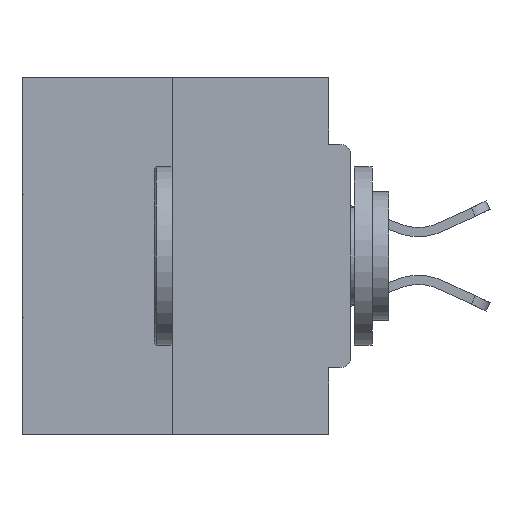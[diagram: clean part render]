
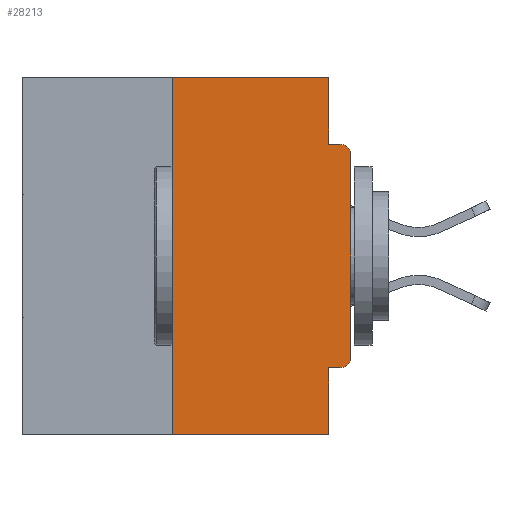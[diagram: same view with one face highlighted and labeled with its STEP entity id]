
A CAD part, left-side view. The second image highlights one B-rep face of the part: STEP entity #28213.
In plain terms, the highlighted planar face has unit normal (-1, 0, 0).
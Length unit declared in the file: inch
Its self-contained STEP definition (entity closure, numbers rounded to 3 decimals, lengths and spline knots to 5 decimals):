
#609 = VERTEX_POINT ( 'NONE', #28277 ) ;
#995 = LINE ( 'NONE', #14118, #32650 ) ;
#1202 = ORIENTED_EDGE ( 'NONE', *, *, #29794, .T. ) ;
#1349 = ORIENTED_EDGE ( 'NONE', *, *, #2727, .T. ) ;
#1656 = LINE ( 'NONE', #17639, #36566 ) ;
#1815 = CARTESIAN_POINT ( 'NONE',  ( 0., 0.25, 0. ) ) ;
#2324 = CARTESIAN_POINT ( 'NONE',  ( 0., 0.015, -0.4065 ) ) ;
#2508 = PLANE ( 'NONE',  #12070 ) ;
#2518 = VERTEX_POINT ( 'NONE', #1815 ) ;
#2727 = EDGE_CURVE ( 'NONE', #4760, #6641, #4569, .T. ) ;
#2770 = CARTESIAN_POINT ( 'NONE',  ( 0., 0.46, 0. ) ) ;
#3148 = CARTESIAN_POINT ( 'NONE',  ( 0., 0.031, -0.5 ) ) ;
#3369 = ORIENTED_EDGE ( 'NONE', *, *, #11654, .F. ) ;
#3539 = EDGE_CURVE ( 'NONE', #609, #2518, #18900, .T. ) ;
#4006 = EDGE_CURVE ( 'NONE', #2518, #28657, #28773, .T. ) ;
#4053 = FACE_OUTER_BOUND ( 'NONE', #20403, .T. ) ;
#4188 = VERTEX_POINT ( 'NONE', #2324 ) ;
#4569 = LINE ( 'NONE', #11789, #25343 ) ;
#4718 = VECTOR ( 'NONE', #10609, 39.37008 ) ;
#4760 = VERTEX_POINT ( 'NONE', #9687 ) ;
#5119 = AXIS2_PLACEMENT_3D ( 'NONE', #16255, #26266, #29038 ) ;
#5538 = CARTESIAN_POINT ( 'NONE',  ( 0., 0., -0.1085 ) ) ;
#5791 = DIRECTION ( 'NONE',  ( 0., 0., -1. ) ) ;
#6390 = ORIENTED_EDGE ( 'NONE', *, *, #3539, .F. ) ;
#6641 = VERTEX_POINT ( 'NONE', #5538 ) ;
#6953 = CARTESIAN_POINT ( 'NONE',  ( 0., 0., -0.4065 ) ) ;
#7112 = CARTESIAN_POINT ( 'NONE',  ( 0., 0.031, -0.0935 ) ) ;
#7282 = EDGE_CURVE ( 'NONE', #17510, #15168, #24228, .T. ) ;
#7765 = ORIENTED_EDGE ( 'NONE', *, *, #7282, .F. ) ;
#8094 = CARTESIAN_POINT ( 'NONE',  ( 0., 0.031, -0.4065 ) ) ;
#9460 = ORIENTED_EDGE ( 'NONE', *, *, #34226, .T. ) ;
#9653 = CIRCLE ( 'NONE', #34637, 0.015 ) ;
#9687 = CARTESIAN_POINT ( 'NONE',  ( 0., 0., -0.3915 ) ) ;
#10094 = CARTESIAN_POINT ( 'NONE',  ( 0., 0.031, 0. ) ) ;
#10609 = DIRECTION ( 'NONE',  ( 0., 1., 0. ) ) ;
#10662 = CARTESIAN_POINT ( 'NONE',  ( 0., 0.25, 0. ) ) ;
#10857 = VECTOR ( 'NONE', #37729, 39.37008 ) ;
#10903 = ORIENTED_EDGE ( 'NONE', *, *, #25022, .T. ) ;
#11654 = EDGE_CURVE ( 'NONE', #28657, #33038, #1656, .T. ) ;
#11789 = CARTESIAN_POINT ( 'NONE',  ( 0., 0., 0. ) ) ;
#12070 = AXIS2_PLACEMENT_3D ( 'NONE', #2770, #30074, #5791 ) ;
#12826 = ORIENTED_EDGE ( 'NONE', *, *, #4006, .F. ) ;
#14005 = EDGE_CURVE ( 'NONE', #4188, #17510, #17926, .T. ) ;
#14118 = CARTESIAN_POINT ( 'NONE',  ( 0., 0.46, -0.5 ) ) ;
#14669 = EDGE_CURVE ( 'NONE', #33038, #22578, #35362, .T. ) ;
#15149 = DIRECTION ( 'NONE',  ( 0., 0., -1. ) ) ;
#15168 = VERTEX_POINT ( 'NONE', #3148 ) ;
#15752 = VECTOR ( 'NONE', #28158, 39.37008 ) ;
#16255 = CARTESIAN_POINT ( 'NONE',  ( 0., 0.015, -0.3915 ) ) ;
#17510 = VERTEX_POINT ( 'NONE', #8094 ) ;
#17639 = CARTESIAN_POINT ( 'NONE',  ( 0., 0.031, 0. ) ) ;
#17926 = LINE ( 'NONE', #6953, #4718 ) ;
#18007 = ORIENTED_EDGE ( 'NONE', *, *, #14005, .F. ) ;
#18682 = CARTESIAN_POINT ( 'NONE',  ( 0., 0.46, 0. ) ) ;
#18900 = LINE ( 'NONE', #10662, #10857 ) ;
#19087 = DIRECTION ( 'NONE',  ( 0., 0., -1. ) ) ;
#19306 = CARTESIAN_POINT ( 'NONE',  ( 0., 0.031, -0.5 ) ) ;
#20403 = EDGE_LOOP ( 'NONE', ( #12826, #6390, #10903, #7765, #18007, #9460, #1349, #1202, #35056, #3369 ) ) ;
#20657 = CARTESIAN_POINT ( 'NONE',  ( 0., 0.015, -0.0935 ) ) ;
#22578 = VERTEX_POINT ( 'NONE', #20657 ) ;
#24228 = LINE ( 'NONE', #19306, #15752 ) ;
#25022 = EDGE_CURVE ( 'NONE', #609, #15168, #995, .T. ) ;
#25343 = VECTOR ( 'NONE', #38997, 39.37008 ) ;
#26266 = DIRECTION ( 'NONE',  ( -1., 0., 0. ) ) ;
#28002 = DIRECTION ( 'NONE',  ( 0., -1., 0. ) ) ;
#28060 = CARTESIAN_POINT ( 'NONE',  ( 0., 0.015, -0.1085 ) ) ;
#28158 = DIRECTION ( 'NONE',  ( 0., 0., -1. ) ) ;
#28213 = ADVANCED_FACE ( 'NONE', ( #4053 ), #2508, .F. ) ;
#28277 = CARTESIAN_POINT ( 'NONE',  ( 0., 0.25, -0.5 ) ) ;
#28657 = VERTEX_POINT ( 'NONE', #10094 ) ;
#28773 = LINE ( 'NONE', #18682, #30212 ) ;
#29038 = DIRECTION ( 'NONE',  ( 0., 0., -1. ) ) ;
#29794 = EDGE_CURVE ( 'NONE', #6641, #22578, #9653, .T. ) ;
#30074 = DIRECTION ( 'NONE',  ( 1., 0., 0. ) ) ;
#30212 = VECTOR ( 'NONE', #31008, 39.37008 ) ;
#31008 = DIRECTION ( 'NONE',  ( 0., -1., 0. ) ) ;
#31351 = CARTESIAN_POINT ( 'NONE',  ( 0., 0., -0.0935 ) ) ;
#32650 = VECTOR ( 'NONE', #38140, 39.37008 ) ;
#33038 = VERTEX_POINT ( 'NONE', #7112 ) ;
#33442 = CIRCLE ( 'NONE', #5119, 0.015 ) ;
#34226 = EDGE_CURVE ( 'NONE', #4188, #4760, #33442, .T. ) ;
#34637 = AXIS2_PLACEMENT_3D ( 'NONE', #28060, #37162, #19087 ) ;
#34924 = VECTOR ( 'NONE', #28002, 39.37008 ) ;
#35056 = ORIENTED_EDGE ( 'NONE', *, *, #14669, .F. ) ;
#35362 = LINE ( 'NONE', #31351, #34924 ) ;
#36566 = VECTOR ( 'NONE', #15149, 39.37008 ) ;
#37162 = DIRECTION ( 'NONE',  ( -1., 0., 0. ) ) ;
#37729 = DIRECTION ( 'NONE',  ( 0., 0., 1. ) ) ;
#38140 = DIRECTION ( 'NONE',  ( 0., -1., 0. ) ) ;
#38997 = DIRECTION ( 'NONE',  ( 0., 0., 1. ) ) ;
